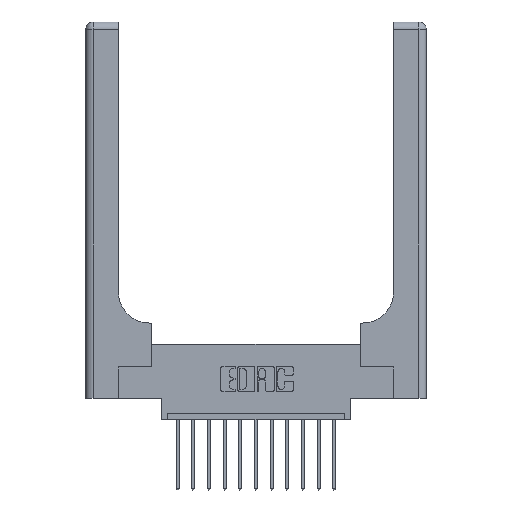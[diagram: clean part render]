
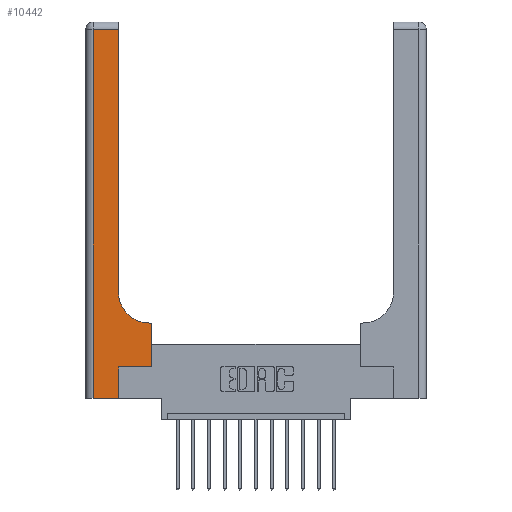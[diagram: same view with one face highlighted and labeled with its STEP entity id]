
A CAD part, top view. The second image highlights one B-rep face of the part: STEP entity #10442.
In plain terms, the highlighted planar face has unit normal (0, 0, 1).
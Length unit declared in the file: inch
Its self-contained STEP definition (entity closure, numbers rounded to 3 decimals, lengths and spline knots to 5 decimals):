
#68 = ORIENTED_EDGE ( 'NONE', *, *, #13909, .T. ) ;
#281 = CARTESIAN_POINT ( 'NONE',  ( 0.51, 0.6, 0.37 ) ) ;
#353 = DIRECTION ( 'NONE',  ( 0., -1., 0. ) ) ;
#522 = CIRCLE ( 'NONE', #9150, 0.25 ) ;
#531 = CARTESIAN_POINT ( 'NONE',  ( 0.06, 3., 0.37 ) ) ;
#982 = EDGE_CURVE ( 'NONE', #4392, #4294, #4554, .T. ) ;
#1288 = EDGE_CURVE ( 'NONE', #3148, #6492, #15206, .T. ) ;
#1606 = VECTOR ( 'NONE', #13866, 39.37008 ) ;
#1691 = LINE ( 'NONE', #13471, #1782 ) ;
#1782 = VECTOR ( 'NONE', #12024, 39.37008 ) ;
#2001 = DIRECTION ( 'NONE',  ( 0., 1., 0. ) ) ;
#2186 = LINE ( 'NONE', #12673, #1606 ) ;
#2358 = VERTEX_POINT ( 'NONE', #8008 ) ;
#3148 = VERTEX_POINT ( 'NONE', #4323 ) ;
#3780 = DIRECTION ( 'NONE',  ( 1., 0., 0. ) ) ;
#3879 = VECTOR ( 'NONE', #2001, 39.37008 ) ;
#3995 = DIRECTION ( 'NONE',  ( -1., 0., 0. ) ) ;
#4050 = ORIENTED_EDGE ( 'NONE', *, *, #14688, .T. ) ;
#4073 = VERTEX_POINT ( 'NONE', #281 ) ;
#4294 = VERTEX_POINT ( 'NONE', #10337 ) ;
#4323 = CARTESIAN_POINT ( 'NONE',  ( 0.528, 0.25, 0.37 ) ) ;
#4392 = VERTEX_POINT ( 'NONE', #9485 ) ;
#4554 = LINE ( 'NONE', #16333, #5220 ) ;
#4583 = DIRECTION ( 'NONE',  ( -1., 0., 0. ) ) ;
#4858 = CARTESIAN_POINT ( 'NONE',  ( 0., 3., 0.37 ) ) ;
#4937 = CARTESIAN_POINT ( 'NONE',  ( 0.26, 0.85, 0.37 ) ) ;
#5220 = VECTOR ( 'NONE', #11089, 39.37008 ) ;
#5272 = LINE ( 'NONE', #5440, #6589 ) ;
#5343 = CARTESIAN_POINT ( 'NONE',  ( 0.06, 2.94, 0.37 ) ) ;
#5440 = CARTESIAN_POINT ( 'NONE',  ( 0.26, 0.6, 0.37 ) ) ;
#5598 = ORIENTED_EDGE ( 'NONE', *, *, #6794, .T. ) ;
#5867 = CARTESIAN_POINT ( 'NONE',  ( 0., 2.94, 0.37 ) ) ;
#5895 = CARTESIAN_POINT ( 'NONE',  ( 0.528, 0.25, 0.37 ) ) ;
#6162 = EDGE_CURVE ( 'NONE', #6492, #4073, #5272, .T. ) ;
#6492 = VERTEX_POINT ( 'NONE', #10497 ) ;
#6589 = VECTOR ( 'NONE', #3995, 39.37008 ) ;
#6794 = EDGE_CURVE ( 'NONE', #4294, #3148, #1691, .T. ) ;
#7914 = CARTESIAN_POINT ( 'NONE',  ( 0.51, 0.85, 0.37 ) ) ;
#8008 = CARTESIAN_POINT ( 'NONE',  ( 0.06, 0., 0.37 ) ) ;
#8198 = EDGE_CURVE ( 'NONE', #2358, #4392, #2186, .T. ) ;
#8517 = EDGE_CURVE ( 'NONE', #4073, #9325, #522, .T. ) ;
#8746 = DIRECTION ( 'NONE',  ( -1., 0., 0. ) ) ;
#9150 = AXIS2_PLACEMENT_3D ( 'NONE', #7914, #13089, #3780 ) ;
#9325 = VERTEX_POINT ( 'NONE', #4937 ) ;
#9401 = EDGE_CURVE ( 'NONE', #12287, #2358, #14510, .T. ) ;
#9485 = CARTESIAN_POINT ( 'NONE',  ( 0.265, 0., 0.37 ) ) ;
#9766 = FACE_OUTER_BOUND ( 'NONE', #9906, .T. ) ;
#9874 = ORIENTED_EDGE ( 'NONE', *, *, #9401, .T. ) ;
#9906 = EDGE_LOOP ( 'NONE', ( #68, #4050, #9874, #11612, #11284, #5598, #10745, #12501, #9991 ) ) ;
#9991 = ORIENTED_EDGE ( 'NONE', *, *, #8517, .T. ) ;
#10337 = CARTESIAN_POINT ( 'NONE',  ( 0.265, 0.25, 0.37 ) ) ;
#10442 = ADVANCED_FACE ( 'NONE', ( #9766 ), #16474, .F. ) ;
#10497 = CARTESIAN_POINT ( 'NONE',  ( 0.528, 0.6, 0.37 ) ) ;
#10745 = ORIENTED_EDGE ( 'NONE', *, *, #1288, .T. ) ;
#11089 = DIRECTION ( 'NONE',  ( 0., 1., 0. ) ) ;
#11156 = CARTESIAN_POINT ( 'NONE',  ( 0.26, 3., 0.37 ) ) ;
#11284 = ORIENTED_EDGE ( 'NONE', *, *, #982, .T. ) ;
#11612 = ORIENTED_EDGE ( 'NONE', *, *, #8198, .T. ) ;
#11918 = VECTOR ( 'NONE', #16320, 39.37008 ) ;
#12018 = LINE ( 'NONE', #11156, #11918 ) ;
#12024 = DIRECTION ( 'NONE',  ( 1., 0., 0. ) ) ;
#12287 = VERTEX_POINT ( 'NONE', #5343 ) ;
#12501 = ORIENTED_EDGE ( 'NONE', *, *, #6162, .T. ) ;
#12673 = CARTESIAN_POINT ( 'NONE',  ( 0., 0., 0.37 ) ) ;
#12794 = CARTESIAN_POINT ( 'NONE',  ( 0.26, 2.94, 0.37 ) ) ;
#13089 = DIRECTION ( 'NONE',  ( 0., 0., -1. ) ) ;
#13471 = CARTESIAN_POINT ( 'NONE',  ( 0.265, 0.25, 0.37 ) ) ;
#13843 = VECTOR ( 'NONE', #4583, 39.37008 ) ;
#13866 = DIRECTION ( 'NONE',  ( 1., 0., 0. ) ) ;
#13909 = EDGE_CURVE ( 'NONE', #9325, #15922, #12018, .T. ) ;
#14510 = LINE ( 'NONE', #531, #16776 ) ;
#14688 = EDGE_CURVE ( 'NONE', #15922, #12287, #16199, .T. ) ;
#15114 = AXIS2_PLACEMENT_3D ( 'NONE', #4858, #15200, #8746 ) ;
#15200 = DIRECTION ( 'NONE',  ( 0., 0., -1. ) ) ;
#15206 = LINE ( 'NONE', #5895, #3879 ) ;
#15922 = VERTEX_POINT ( 'NONE', #12794 ) ;
#16199 = LINE ( 'NONE', #5867, #13843 ) ;
#16320 = DIRECTION ( 'NONE',  ( 0., 1., 0. ) ) ;
#16333 = CARTESIAN_POINT ( 'NONE',  ( 0.265, 0., 0.37 ) ) ;
#16474 = PLANE ( 'NONE',  #15114 ) ;
#16776 = VECTOR ( 'NONE', #353, 39.37008 ) ;
